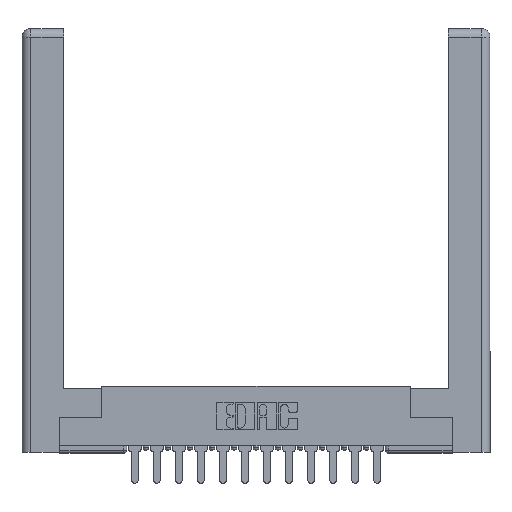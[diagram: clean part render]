
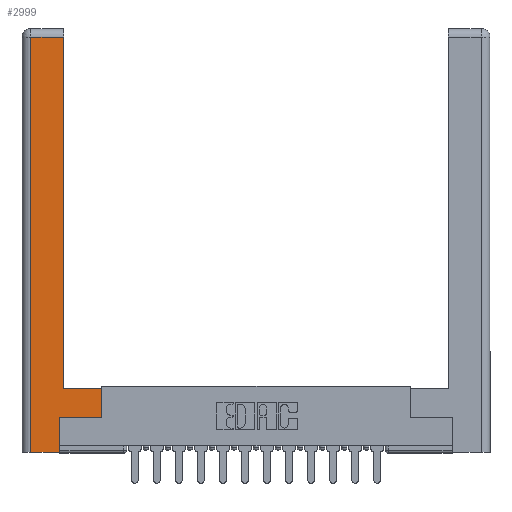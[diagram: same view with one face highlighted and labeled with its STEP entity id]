
A CAD part, top view. The second image highlights one B-rep face of the part: STEP entity #2999.
In plain terms, the highlighted planar face has unit normal (0, 0, 1).
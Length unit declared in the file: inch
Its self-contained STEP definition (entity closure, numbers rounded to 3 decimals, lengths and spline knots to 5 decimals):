
#669 = EDGE_LOOP ( 'NONE', ( #2532, #13132, #6715, #2089, #9298, #8129, #8440, #1842 ) ) ;
#1136 = DIRECTION ( 'NONE',  ( 0., 1., 0. ) ) ;
#1379 = EDGE_CURVE ( 'NONE', #9218, #3509, #6378, .T. ) ;
#1842 = ORIENTED_EDGE ( 'NONE', *, *, #13992, .T. ) ;
#1975 = DIRECTION ( 'NONE',  ( -1., 0., 0. ) ) ;
#2012 = CARTESIAN_POINT ( 'NONE',  ( 0.0615, 0., 0. ) ) ;
#2039 = CARTESIAN_POINT ( 'NONE',  ( 0.0615, 2.94, 0. ) ) ;
#2089 = ORIENTED_EDGE ( 'NONE', *, *, #6427, .T. ) ;
#2176 = LINE ( 'NONE', #16414, #5762 ) ;
#2532 = ORIENTED_EDGE ( 'NONE', *, *, #1379, .T. ) ;
#2782 = EDGE_CURVE ( 'NONE', #9026, #9692, #14350, .T. ) ;
#2999 = ADVANCED_FACE ( 'NONE', ( #16352 ), #5747, .F. ) ;
#3509 = VERTEX_POINT ( 'NONE', #5085 ) ;
#3735 = VERTEX_POINT ( 'NONE', #14901 ) ;
#4099 = EDGE_CURVE ( 'NONE', #4751, #9026, #7288, .T. ) ;
#4182 = LINE ( 'NONE', #7158, #5186 ) ;
#4751 = VERTEX_POINT ( 'NONE', #12316 ) ;
#5056 = DIRECTION ( 'NONE',  ( 1., 0., 0. ) ) ;
#5085 = CARTESIAN_POINT ( 'NONE',  ( 0.295, 2.94, 0. ) ) ;
#5186 = VECTOR ( 'NONE', #7224, 39.37008 ) ;
#5204 = EDGE_CURVE ( 'NONE', #16404, #10150, #16235, .T. ) ;
#5586 = CARTESIAN_POINT ( 'NONE',  ( 0., 0., 0. ) ) ;
#5747 = PLANE ( 'NONE',  #16579 ) ;
#5762 = VECTOR ( 'NONE', #1136, 39.37008 ) ;
#6378 = LINE ( 'NONE', #8447, #14402 ) ;
#6427 = EDGE_CURVE ( 'NONE', #10150, #4751, #4182, .T. ) ;
#6545 = CARTESIAN_POINT ( 'NONE',  ( 0.565, 0.245, 0. ) ) ;
#6715 = ORIENTED_EDGE ( 'NONE', *, *, #5204, .T. ) ;
#6868 = CARTESIAN_POINT ( 'NONE',  ( 0.0615, 0., 0. ) ) ;
#7094 = VECTOR ( 'NONE', #14022, 39.37008 ) ;
#7158 = CARTESIAN_POINT ( 'NONE',  ( 0.265, 0., 0. ) ) ;
#7187 = CARTESIAN_POINT ( 'NONE',  ( 0.265, 0.245, 0. ) ) ;
#7224 = DIRECTION ( 'NONE',  ( 1., 0., 0. ) ) ;
#7288 = LINE ( 'NONE', #9857, #14893 ) ;
#8129 = ORIENTED_EDGE ( 'NONE', *, *, #2782, .T. ) ;
#8401 = EDGE_CURVE ( 'NONE', #9692, #3735, #2176, .T. ) ;
#8440 = ORIENTED_EDGE ( 'NONE', *, *, #8401, .T. ) ;
#8447 = CARTESIAN_POINT ( 'NONE',  ( 0.295, 3., 0. ) ) ;
#9026 = VERTEX_POINT ( 'NONE', #7187 ) ;
#9218 = VERTEX_POINT ( 'NONE', #15144 ) ;
#9298 = ORIENTED_EDGE ( 'NONE', *, *, #4099, .T. ) ;
#9496 = LINE ( 'NONE', #14068, #7094 ) ;
#9682 = EDGE_CURVE ( 'NONE', #3509, #16404, #10741, .T. ) ;
#9692 = VERTEX_POINT ( 'NONE', #12559 ) ;
#9857 = CARTESIAN_POINT ( 'NONE',  ( 0.265, 0.245, 0. ) ) ;
#9973 = DIRECTION ( 'NONE',  ( 0., 1., 0. ) ) ;
#10150 = VERTEX_POINT ( 'NONE', #6868 ) ;
#10741 = LINE ( 'NONE', #2039, #15157 ) ;
#12316 = CARTESIAN_POINT ( 'NONE',  ( 0.265, 0., 0. ) ) ;
#12559 = CARTESIAN_POINT ( 'NONE',  ( 0.565, 0.245, 0. ) ) ;
#13132 = ORIENTED_EDGE ( 'NONE', *, *, #9682, .T. ) ;
#13489 = DIRECTION ( 'NONE',  ( 0., 0., -1. ) ) ;
#13657 = DIRECTION ( 'NONE',  ( -1., 0., 0. ) ) ;
#13992 = EDGE_CURVE ( 'NONE', #3735, #9218, #9496, .T. ) ;
#14022 = DIRECTION ( 'NONE',  ( -1., 0., 0. ) ) ;
#14068 = CARTESIAN_POINT ( 'NONE',  ( 0.295, 0.45, 0. ) ) ;
#14069 = CARTESIAN_POINT ( 'NONE',  ( 0.0615, 2.94, 0. ) ) ;
#14350 = LINE ( 'NONE', #6545, #16158 ) ;
#14402 = VECTOR ( 'NONE', #14666, 39.37008 ) ;
#14615 = VECTOR ( 'NONE', #15941, 39.37008 ) ;
#14666 = DIRECTION ( 'NONE',  ( 0., 1., 0. ) ) ;
#14893 = VECTOR ( 'NONE', #9973, 39.37008 ) ;
#14901 = CARTESIAN_POINT ( 'NONE',  ( 0.565, 0.45, 0. ) ) ;
#15144 = CARTESIAN_POINT ( 'NONE',  ( 0.295, 0.45, 0. ) ) ;
#15157 = VECTOR ( 'NONE', #13657, 39.37008 ) ;
#15941 = DIRECTION ( 'NONE',  ( 0., -1., 0. ) ) ;
#16158 = VECTOR ( 'NONE', #5056, 39.37008 ) ;
#16235 = LINE ( 'NONE', #2012, #14615 ) ;
#16352 = FACE_OUTER_BOUND ( 'NONE', #669, .T. ) ;
#16404 = VERTEX_POINT ( 'NONE', #14069 ) ;
#16414 = CARTESIAN_POINT ( 'NONE',  ( 0.565, 0.45, 0. ) ) ;
#16579 = AXIS2_PLACEMENT_3D ( 'NONE', #5586, #13489, #1975 ) ;
